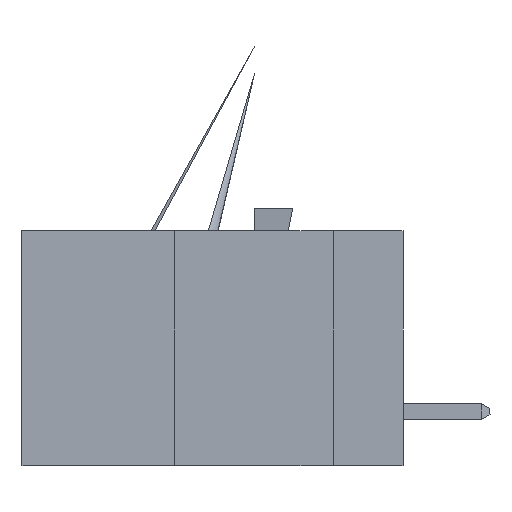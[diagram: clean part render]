
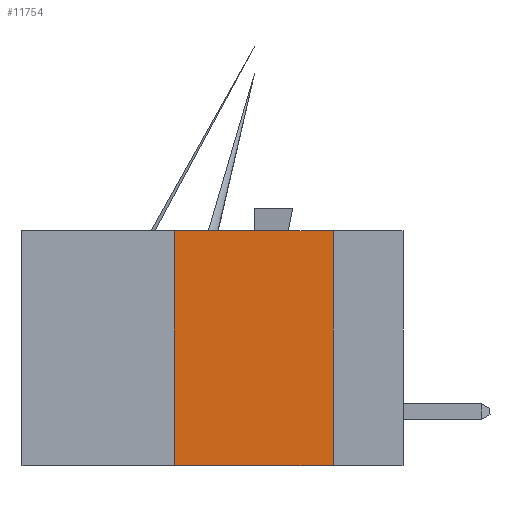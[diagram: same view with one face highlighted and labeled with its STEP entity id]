
A CAD part, left-side view. The second image highlights one B-rep face of the part: STEP entity #11754.
In plain terms, the highlighted planar face has unit normal (-1, 0, 0).
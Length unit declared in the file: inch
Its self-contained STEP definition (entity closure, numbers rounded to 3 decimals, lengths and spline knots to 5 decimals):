
#84 = EDGE_CURVE ( 'NONE', #5659, #9163, #9307, .T. ) ;
#395 = EDGE_CURVE ( 'NONE', #5659, #4810, #6883, .T. ) ;
#1471 = LINE ( 'NONE', #4752, #8893 ) ;
#1830 = CARTESIAN_POINT ( 'NONE',  ( 0., 0.36, 0. ) ) ;
#1850 = CARTESIAN_POINT ( 'NONE',  ( 0., 0.11, 0. ) ) ;
#2301 = VECTOR ( 'NONE', #6582, 39.37008 ) ;
#2334 = DIRECTION ( 'NONE',  ( 0., -1., 0. ) ) ;
#2627 = DIRECTION ( 'NONE',  ( 1., 0., 0. ) ) ;
#4379 = VECTOR ( 'NONE', #2334, 39.37008 ) ;
#4505 = PLANE ( 'NONE',  #8597 ) ;
#4528 = CARTESIAN_POINT ( 'NONE',  ( 0., 0.11, 0. ) ) ;
#4752 = CARTESIAN_POINT ( 'NONE',  ( 0., 0.6, 0. ) ) ;
#4772 = EDGE_CURVE ( 'NONE', #10638, #4810, #9032, .T. ) ;
#4810 = VERTEX_POINT ( 'NONE', #9277 ) ;
#4941 = ORIENTED_EDGE ( 'NONE', *, *, #4772, .F. ) ;
#4989 = CARTESIAN_POINT ( 'NONE',  ( 0., 0.6, -0.37 ) ) ;
#5111 = FACE_OUTER_BOUND ( 'NONE', #8302, .T. ) ;
#5432 = EDGE_CURVE ( 'NONE', #9163, #10638, #1471, .T. ) ;
#5551 = ORIENTED_EDGE ( 'NONE', *, *, #395, .T. ) ;
#5659 = VERTEX_POINT ( 'NONE', #11154 ) ;
#5710 = DIRECTION ( 'NONE',  ( 0., -1., 0. ) ) ;
#6582 = DIRECTION ( 'NONE',  ( 0., 0., 1. ) ) ;
#6883 = LINE ( 'NONE', #4989, #4379 ) ;
#6959 = CARTESIAN_POINT ( 'NONE',  ( 0., 0.36, 0. ) ) ;
#8173 = CARTESIAN_POINT ( 'NONE',  ( 0., 0.6, 0. ) ) ;
#8302 = EDGE_LOOP ( 'NONE', ( #4941, #11930, #9963, #5551 ) ) ;
#8383 = DIRECTION ( 'NONE',  ( 0., 0., -1. ) ) ;
#8597 = AXIS2_PLACEMENT_3D ( 'NONE', #8173, #2627, #9048 ) ;
#8768 = VECTOR ( 'NONE', #8383, 39.37008 ) ;
#8893 = VECTOR ( 'NONE', #5710, 39.37008 ) ;
#9032 = LINE ( 'NONE', #1850, #8768 ) ;
#9048 = DIRECTION ( 'NONE',  ( 0., 0., -1. ) ) ;
#9163 = VERTEX_POINT ( 'NONE', #6959 ) ;
#9277 = CARTESIAN_POINT ( 'NONE',  ( 0., 0.11, -0.37 ) ) ;
#9307 = LINE ( 'NONE', #1830, #2301 ) ;
#9963 = ORIENTED_EDGE ( 'NONE', *, *, #84, .F. ) ;
#10638 = VERTEX_POINT ( 'NONE', #4528 ) ;
#11154 = CARTESIAN_POINT ( 'NONE',  ( 0., 0.36, -0.37 ) ) ;
#11754 = ADVANCED_FACE ( 'NONE', ( #5111 ), #4505, .F. ) ;
#11930 = ORIENTED_EDGE ( 'NONE', *, *, #5432, .F. ) ;
